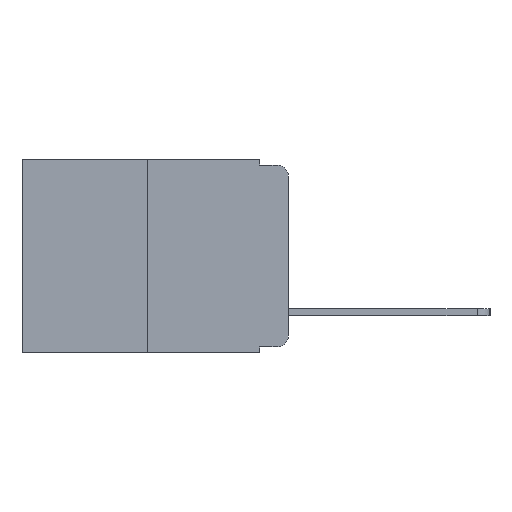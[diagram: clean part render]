
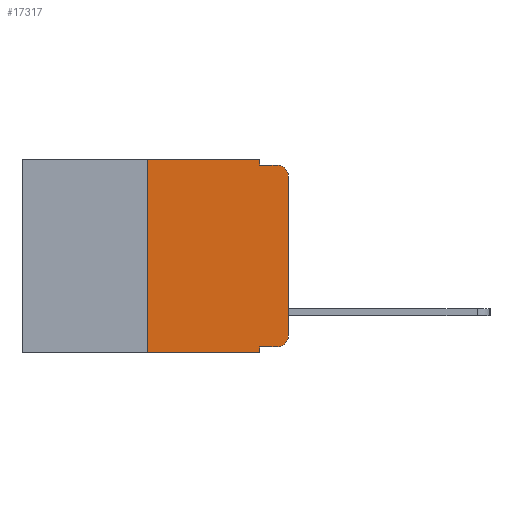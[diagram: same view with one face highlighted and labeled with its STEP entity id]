
A CAD part, left-side view. The second image highlights one B-rep face of the part: STEP entity #17317.
In plain terms, the highlighted planar face has unit normal (-1, 0, 0).
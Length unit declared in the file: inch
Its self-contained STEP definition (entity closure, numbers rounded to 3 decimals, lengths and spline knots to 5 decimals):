
#440 = VECTOR ( 'NONE', #10553, 39.37008 ) ;
#730 = EDGE_CURVE ( 'NONE', #2890, #2541, #8619, .T. ) ;
#1229 = ORIENTED_EDGE ( 'NONE', *, *, #14497, .T. ) ;
#1258 = ORIENTED_EDGE ( 'NONE', *, *, #15592, .F. ) ;
#1277 = EDGE_CURVE ( 'NONE', #7009, #22842, #2058, .T. ) ;
#2058 = LINE ( 'NONE', #10745, #2685 ) ;
#2541 = VERTEX_POINT ( 'NONE', #15822 ) ;
#2578 = CARTESIAN_POINT ( 'NONE',  ( 0., 0.051, -0.343 ) ) ;
#2685 = VECTOR ( 'NONE', #22773, 39.37008 ) ;
#2890 = VERTEX_POINT ( 'NONE', #20095 ) ;
#3140 = LINE ( 'NONE', #21302, #6792 ) ;
#3366 = AXIS2_PLACEMENT_3D ( 'NONE', #6043, #18248, #7861 ) ;
#3751 = ORIENTED_EDGE ( 'NONE', *, *, #10087, .T. ) ;
#3877 = VECTOR ( 'NONE', #12568, 39.37008 ) ;
#4118 = CARTESIAN_POINT ( 'NONE',  ( 0., 0.02, -0.313 ) ) ;
#4463 = CARTESIAN_POINT ( 'NONE',  ( 0., 0., -0.03 ) ) ;
#4607 = PLANE ( 'NONE',  #18695 ) ;
#4854 = ORIENTED_EDGE ( 'NONE', *, *, #5040, .T. ) ;
#4935 = LINE ( 'NONE', #18594, #13232 ) ;
#5040 = EDGE_CURVE ( 'NONE', #22842, #11963, #17920, .T. ) ;
#5465 = LINE ( 'NONE', #20877, #440 ) ;
#5864 = CARTESIAN_POINT ( 'NONE',  ( 0., 0.02, -0.333 ) ) ;
#5946 = DIRECTION ( 'NONE',  ( 0., 0., -1. ) ) ;
#5952 = LINE ( 'NONE', #6684, #19834 ) ;
#6043 = CARTESIAN_POINT ( 'NONE',  ( 0., 0.02, -0.03 ) ) ;
#6554 = CIRCLE ( 'NONE', #15559, 0.02 ) ;
#6625 = LINE ( 'NONE', #20504, #15921 ) ;
#6684 = CARTESIAN_POINT ( 'NONE',  ( 0., 0.051, -0.333 ) ) ;
#6792 = VECTOR ( 'NONE', #12752, 39.37008 ) ;
#7009 = VERTEX_POINT ( 'NONE', #16076 ) ;
#7425 = VERTEX_POINT ( 'NONE', #15468 ) ;
#7646 = ORIENTED_EDGE ( 'NONE', *, *, #1277, .T. ) ;
#7861 = DIRECTION ( 'NONE',  ( 0., 0., -1. ) ) ;
#8087 = VECTOR ( 'NONE', #10911, 39.37008 ) ;
#8182 = ORIENTED_EDGE ( 'NONE', *, *, #16735, .F. ) ;
#8229 = DIRECTION ( 'NONE',  ( 1., 0., 0. ) ) ;
#8521 = VERTEX_POINT ( 'NONE', #2578 ) ;
#8619 = LINE ( 'NONE', #17785, #8087 ) ;
#8837 = ORIENTED_EDGE ( 'NONE', *, *, #10953, .T. ) ;
#9837 = ORIENTED_EDGE ( 'NONE', *, *, #22497, .F. ) ;
#9974 = VERTEX_POINT ( 'NONE', #12674 ) ;
#10087 = EDGE_CURVE ( 'NONE', #21475, #7009, #6554, .T. ) ;
#10553 = DIRECTION ( 'NONE',  ( 0., 0., 1. ) ) ;
#10745 = CARTESIAN_POINT ( 'NONE',  ( 0., 0., 0. ) ) ;
#10803 = CARTESIAN_POINT ( 'NONE',  ( 0., 0.051, 0. ) ) ;
#10911 = DIRECTION ( 'NONE',  ( 0., 0., -1. ) ) ;
#10953 = EDGE_CURVE ( 'NONE', #7425, #21475, #5952, .T. ) ;
#11807 = EDGE_LOOP ( 'NONE', ( #7646, #4854, #8182, #13203, #12709, #9837, #1229, #1258, #8837, #3751 ) ) ;
#11963 = VERTEX_POINT ( 'NONE', #14952 ) ;
#12568 = DIRECTION ( 'NONE',  ( 0., 0., -1. ) ) ;
#12674 = CARTESIAN_POINT ( 'NONE',  ( 0., 0.25, -0.343 ) ) ;
#12709 = ORIENTED_EDGE ( 'NONE', *, *, #21672, .F. ) ;
#12752 = DIRECTION ( 'NONE',  ( 0., -1., 0. ) ) ;
#13203 = ORIENTED_EDGE ( 'NONE', *, *, #730, .F. ) ;
#13232 = VECTOR ( 'NONE', #22042, 39.37008 ) ;
#13844 = CARTESIAN_POINT ( 'NONE',  ( 0., 0.25, 0. ) ) ;
#14497 = EDGE_CURVE ( 'NONE', #9974, #8521, #3140, .T. ) ;
#14604 = FACE_OUTER_BOUND ( 'NONE', #11807, .T. ) ;
#14952 = CARTESIAN_POINT ( 'NONE',  ( 0., 0.02, -0.01 ) ) ;
#15331 = DIRECTION ( 'NONE',  ( 0., -1., 0. ) ) ;
#15468 = CARTESIAN_POINT ( 'NONE',  ( 0., 0.051, -0.333 ) ) ;
#15559 = AXIS2_PLACEMENT_3D ( 'NONE', #4118, #16394, #5946 ) ;
#15592 = EDGE_CURVE ( 'NONE', #7425, #8521, #18420, .T. ) ;
#15822 = CARTESIAN_POINT ( 'NONE',  ( 0., 0.051, -0.01 ) ) ;
#15921 = VECTOR ( 'NONE', #15331, 39.37008 ) ;
#16076 = CARTESIAN_POINT ( 'NONE',  ( 0., 0., -0.313 ) ) ;
#16394 = DIRECTION ( 'NONE',  ( -1., 0., 0. ) ) ;
#16735 = EDGE_CURVE ( 'NONE', #2541, #11963, #6625, .T. ) ;
#16857 = CARTESIAN_POINT ( 'NONE',  ( 0., 0.473, 0. ) ) ;
#17113 = DIRECTION ( 'NONE',  ( 0., -1., 0. ) ) ;
#17317 = ADVANCED_FACE ( 'NONE', ( #14604 ), #4607, .F. ) ;
#17785 = CARTESIAN_POINT ( 'NONE',  ( 0., 0.051, 0. ) ) ;
#17920 = CIRCLE ( 'NONE', #3366, 0.02 ) ;
#18248 = DIRECTION ( 'NONE',  ( -1., 0., 0. ) ) ;
#18420 = LINE ( 'NONE', #10803, #3877 ) ;
#18594 = CARTESIAN_POINT ( 'NONE',  ( 0., 0.473, 0. ) ) ;
#18695 = AXIS2_PLACEMENT_3D ( 'NONE', #16857, #8229, #20337 ) ;
#19834 = VECTOR ( 'NONE', #17113, 39.37008 ) ;
#20095 = CARTESIAN_POINT ( 'NONE',  ( 0., 0.051, 0. ) ) ;
#20337 = DIRECTION ( 'NONE',  ( 0., 0., -1. ) ) ;
#20504 = CARTESIAN_POINT ( 'NONE',  ( 0., 0.051, -0.01 ) ) ;
#20587 = VERTEX_POINT ( 'NONE', #13844 ) ;
#20877 = CARTESIAN_POINT ( 'NONE',  ( 0., 0.25, 0. ) ) ;
#21302 = CARTESIAN_POINT ( 'NONE',  ( 0., 0.473, -0.343 ) ) ;
#21475 = VERTEX_POINT ( 'NONE', #5864 ) ;
#21672 = EDGE_CURVE ( 'NONE', #20587, #2890, #4935, .T. ) ;
#22042 = DIRECTION ( 'NONE',  ( 0., -1., 0. ) ) ;
#22497 = EDGE_CURVE ( 'NONE', #9974, #20587, #5465, .T. ) ;
#22773 = DIRECTION ( 'NONE',  ( 0., 0., 1. ) ) ;
#22842 = VERTEX_POINT ( 'NONE', #4463 ) ;
